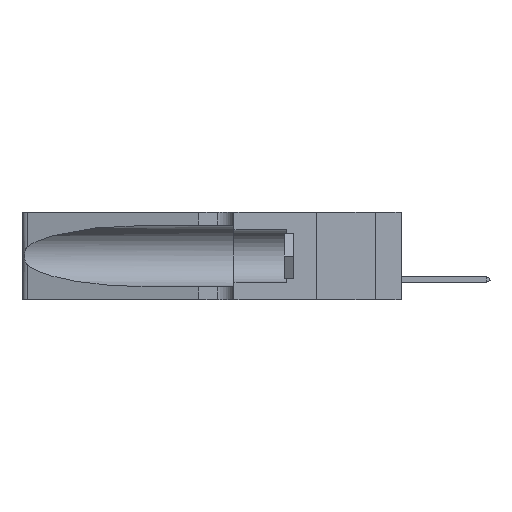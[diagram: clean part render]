
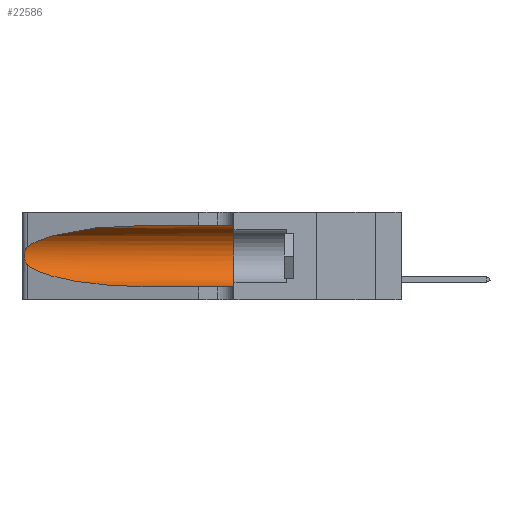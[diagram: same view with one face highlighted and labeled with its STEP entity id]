
A CAD part, left-side view. The second image highlights one B-rep face of the part: STEP entity #22586.
In plain terms, the highlighted cylindrical face has radius 3.308 mm (diameter 6.617 mm), a partial arc.
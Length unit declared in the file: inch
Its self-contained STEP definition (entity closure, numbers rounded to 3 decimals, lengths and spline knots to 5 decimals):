
#431 = VERTEX_POINT ( 'NONE', #25422 ) ;
#874 = LINE ( 'NONE', #15655, #18208 ) ;
#1428 = CARTESIAN_POINT ( 'NONE',  ( 0.25854, 1.2359, 0.20912 ) ) ;
#1446 = CARTESIAN_POINT ( 'NONE',  ( 0.25487, 1.22718, 0.14631 ) ) ;
#1566 =( BOUNDED_CURVE ( )  B_SPLINE_CURVE ( 3, ( #9697, #26293, #18093, #22302 ),
 .UNSPECIFIED., .F., .F. ) 
 B_SPLINE_CURVE_WITH_KNOTS ( ( 4, 4 ),
 ( 3.44316, 4.71239 ),
 .UNSPECIFIED. ) 
 CURVE ( )  GEOMETRIC_REPRESENTATION_ITEM ( )  RATIONAL_B_SPLINE_CURVE ( ( 1., 0.87, 0.87, 1. ) ) 
 REPRESENTATION_ITEM ( '' )  );
#2058 = CARTESIAN_POINT ( 'NONE',  ( 0.1305, 0.35, 0.05475 ) ) ;
#2331 = ORIENTED_EDGE ( 'NONE', *, *, #13368, .F. ) ;
#2365 = B_SPLINE_CURVE_WITH_KNOTS ( 'NONE', 3,
 ( #18098, #11848, #7909, #24228, #1428, #18176, #9703, #13717, #5929, #25931, #21951, #15769, #3513, #17827 ),
 .UNSPECIFIED., .F., .F.,
 ( 4, 2, 2, 2, 2, 2, 4 ),
 ( 0., 0.00027, 0.00053, 0.00107, 0.0016, 0.00187, 0.00214 ),
 .UNSPECIFIED. ) ;
#3328 = EDGE_LOOP ( 'NONE', ( #5911, #12117, #24891, #4134, #2331, #8461 ) ) ;
#3513 = CARTESIAN_POINT ( 'NONE',  ( 0.25555, 1.22993, 0.14849 ) ) ;
#3784 = CARTESIAN_POINT ( 'NONE',  ( 0.1305, 1.61858, 0.05475 ) ) ;
#4134 = ORIENTED_EDGE ( 'NONE', *, *, #16163, .T. ) ;
#4240 = EDGE_CURVE ( 'NONE', #4365, #21547, #1566, .T. ) ;
#4365 = VERTEX_POINT ( 'NONE', #1446 ) ;
#5842 = DIRECTION ( 'NONE',  ( 0., -1., 0. ) ) ;
#5911 = ORIENTED_EDGE ( 'NONE', *, *, #18923, .T. ) ;
#5929 = CARTESIAN_POINT ( 'NONE',  ( 0.26017, 1.23833, 0.17102 ) ) ;
#6700 = DIRECTION ( 'NONE',  ( 0., 0., 1. ) ) ;
#7909 = CARTESIAN_POINT ( 'NONE',  ( 0.25639, 1.23184, 0.21858 ) ) ;
#8086 = CIRCLE ( 'NONE', #14352, 0.13025 ) ;
#8151 = CARTESIAN_POINT ( 'NONE',  ( 0.1305, 0.35, 0.31525 ) ) ;
#8418 = DIRECTION ( 'NONE',  ( 0., -1., 0. ) ) ;
#8461 = ORIENTED_EDGE ( 'NONE', *, *, #25086, .F. ) ;
#8899 = VECTOR ( 'NONE', #5842, 39.37008 ) ;
#9098 = CARTESIAN_POINT ( 'NONE',  ( 0.18966, 0.96281, 0.31525 ) ) ;
#9186 = CARTESIAN_POINT ( 'NONE',  ( 0.1305, 0.72297, 0.31525 ) ) ;
#9697 = CARTESIAN_POINT ( 'NONE',  ( 0.25487, 1.22718, 0.14631 ) ) ;
#9703 = CARTESIAN_POINT ( 'NONE',  ( 0.26075, 1.23896, 0.19203 ) ) ;
#10484 = CARTESIAN_POINT ( 'NONE',  ( 0.1305, 0.72297, 0.05475 ) ) ;
#11848 = CARTESIAN_POINT ( 'NONE',  ( 0.25555, 1.22994, 0.2215 ) ) ;
#12117 = ORIENTED_EDGE ( 'NONE', *, *, #21317, .T. ) ;
#12676 = CYLINDRICAL_SURFACE ( 'NONE', #20364, 0.13025 ) ;
#13368 = EDGE_CURVE ( 'NONE', #21576, #24523, #8086, .T. ) ;
#13717 = CARTESIAN_POINT ( 'NONE',  ( 0.26075, 1.23896, 0.178 ) ) ;
#14352 = AXIS2_PLACEMENT_3D ( 'NONE', #18925, #14921, #6700 ) ;
#14921 = DIRECTION ( 'NONE',  ( 0., 1., 0. ) ) ;
#15655 = CARTESIAN_POINT ( 'NONE',  ( 0.1305, 1.61858, 0.31525 ) ) ;
#15769 = CARTESIAN_POINT ( 'NONE',  ( 0.25639, 1.23186, 0.15144 ) ) ;
#16163 = EDGE_CURVE ( 'NONE', #21547, #24523, #19467, .T. ) ;
#17827 = CARTESIAN_POINT ( 'NONE',  ( 0.25487, 1.22718, 0.14631 ) ) ;
#18093 = CARTESIAN_POINT ( 'NONE',  ( 0.18966, 0.96281, 0.05475 ) ) ;
#18098 = CARTESIAN_POINT ( 'NONE',  ( 0.25487, 1.22718, 0.22369 ) ) ;
#18176 = CARTESIAN_POINT ( 'NONE',  ( 0.26018, 1.23835, 0.19895 ) ) ;
#18208 = VECTOR ( 'NONE', #21921, 39.37008 ) ;
#18923 = EDGE_CURVE ( 'NONE', #19239, #431, #26146, .T. ) ;
#18925 = CARTESIAN_POINT ( 'NONE',  ( 0.1305, 0.35, 0.185 ) ) ;
#18936 = DIRECTION ( 'NONE',  ( 0., 0., -1. ) ) ;
#19239 = VERTEX_POINT ( 'NONE', #23712 ) ;
#19467 = LINE ( 'NONE', #3784, #8899 ) ;
#20364 = AXIS2_PLACEMENT_3D ( 'NONE', #24734, #8418, #18936 ) ;
#21249 = CARTESIAN_POINT ( 'NONE',  ( 0.2373, 1.15595, 0.28018 ) ) ;
#21317 = EDGE_CURVE ( 'NONE', #431, #4365, #2365, .T. ) ;
#21547 = VERTEX_POINT ( 'NONE', #10484 ) ;
#21576 = VERTEX_POINT ( 'NONE', #8151 ) ;
#21921 = DIRECTION ( 'NONE',  ( 0., -1., 0. ) ) ;
#21951 = CARTESIAN_POINT ( 'NONE',  ( 0.25789, 1.23486, 0.15765 ) ) ;
#22302 = CARTESIAN_POINT ( 'NONE',  ( 0.1305, 0.72297, 0.05475 ) ) ;
#22586 = ADVANCED_FACE ( 'NONE', ( #23516 ), #12676, .F. ) ;
#23516 = FACE_OUTER_BOUND ( 'NONE', #3328, .T. ) ;
#23712 = CARTESIAN_POINT ( 'NONE',  ( 0.1305, 0.72297, 0.31525 ) ) ;
#24228 = CARTESIAN_POINT ( 'NONE',  ( 0.25787, 1.23484, 0.2124 ) ) ;
#24523 = VERTEX_POINT ( 'NONE', #2058 ) ;
#24734 = CARTESIAN_POINT ( 'NONE',  ( 0.1305, 1.61858, 0.185 ) ) ;
#24891 = ORIENTED_EDGE ( 'NONE', *, *, #4240, .T. ) ;
#25086 = EDGE_CURVE ( 'NONE', #19239, #21576, #874, .T. ) ;
#25400 = CARTESIAN_POINT ( 'NONE',  ( 0.25487, 1.22718, 0.22369 ) ) ;
#25422 = CARTESIAN_POINT ( 'NONE',  ( 0.25487, 1.22718, 0.22369 ) ) ;
#25931 = CARTESIAN_POINT ( 'NONE',  ( 0.25856, 1.23593, 0.16098 ) ) ;
#26146 =( BOUNDED_CURVE ( )  B_SPLINE_CURVE ( 3, ( #9186, #9098, #21249, #25400 ),
 .UNSPECIFIED., .F., .F. ) 
 B_SPLINE_CURVE_WITH_KNOTS ( ( 4, 4 ),
 ( 1.5708, 2.84003 ),
 .UNSPECIFIED. ) 
 CURVE ( )  GEOMETRIC_REPRESENTATION_ITEM ( )  RATIONAL_B_SPLINE_CURVE ( ( 1., 0.87, 0.87, 1. ) ) 
 REPRESENTATION_ITEM ( '' )  );
#26293 = CARTESIAN_POINT ( 'NONE',  ( 0.2373, 1.15595, 0.08982 ) ) ;
